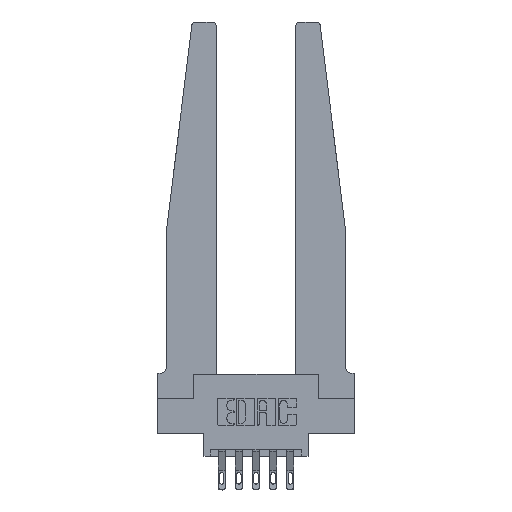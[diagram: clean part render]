
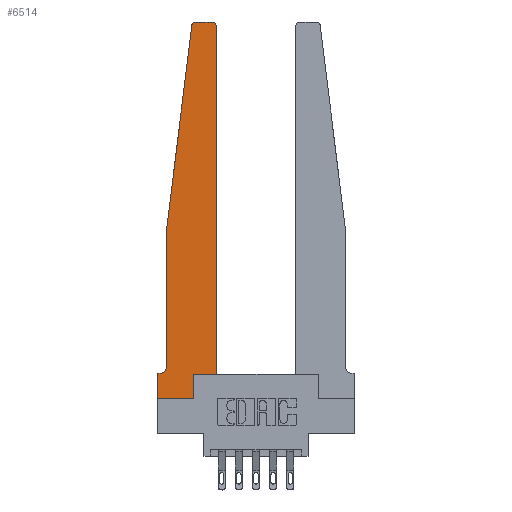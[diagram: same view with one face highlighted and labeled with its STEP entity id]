
A CAD part, top view. The second image highlights one B-rep face of the part: STEP entity #6514.
In plain terms, the highlighted planar face has unit normal (0, 0, 1).
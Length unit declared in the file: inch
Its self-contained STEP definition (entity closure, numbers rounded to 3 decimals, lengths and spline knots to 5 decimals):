
#19 = CARTESIAN_POINT ( 'NONE',  ( 0.015, 0.2375, 0.37 ) ) ;
#197 = CARTESIAN_POINT ( 'NONE',  ( 0.395, 2.72, 0.37 ) ) ;
#228 = DIRECTION ( 'NONE',  ( 0., 1., 0. ) ) ;
#386 = CARTESIAN_POINT ( 'NONE',  ( 0., 0., 0.37 ) ) ;
#636 = EDGE_CURVE ( 'NONE', #9752, #9828, #5890, .T. ) ;
#677 = ORIENTED_EDGE ( 'NONE', *, *, #7443, .T. ) ;
#765 = CARTESIAN_POINT ( 'NONE',  ( 0.015, 0.1875, 0.37 ) ) ;
#1002 = DIRECTION ( 'NONE',  ( 0., 0., 1. ) ) ;
#1082 = CARTESIAN_POINT ( 'NONE',  ( 0.395, 2.75, 0.37 ) ) ;
#1124 = DIRECTION ( 'NONE',  ( -1., 0., 0. ) ) ;
#1172 = ORIENTED_EDGE ( 'NONE', *, *, #7420, .T. ) ;
#1224 = EDGE_CURVE ( 'NONE', #6389, #5441, #4889, .T. ) ;
#1286 = CARTESIAN_POINT ( 'NONE',  ( 0., 0., 0.37 ) ) ;
#1292 = DIRECTION ( 'NONE',  ( 1., 0., 0. ) ) ;
#1352 = VERTEX_POINT ( 'NONE', #8733 ) ;
#1486 = DIRECTION ( 'NONE',  ( 1., 0., 0. ) ) ;
#1792 = DIRECTION ( 'NONE',  ( 0., 1., 0. ) ) ;
#1911 = CARTESIAN_POINT ( 'NONE',  ( 0.065, 1.25, 0.37 ) ) ;
#2294 = AXIS2_PLACEMENT_3D ( 'NONE', #197, #7592, #1292 ) ;
#2538 = EDGE_CURVE ( 'NONE', #5441, #6210, #10735, .T. ) ;
#2612 = ORIENTED_EDGE ( 'NONE', *, *, #3065, .T. ) ;
#2754 = EDGE_CURVE ( 'NONE', #3234, #9752, #9168, .T. ) ;
#2767 = LINE ( 'NONE', #7029, #10671 ) ;
#3065 = EDGE_CURVE ( 'NONE', #9119, #3821, #10401, .T. ) ;
#3234 = VERTEX_POINT ( 'NONE', #10200 ) ;
#3355 = ORIENTED_EDGE ( 'NONE', *, *, #2754, .T. ) ;
#3390 = EDGE_CURVE ( 'NONE', #9828, #6389, #12640, .T. ) ;
#3408 = CARTESIAN_POINT ( 'NONE',  ( 0.2605, 0., 0.37 ) ) ;
#3821 = VERTEX_POINT ( 'NONE', #11224 ) ;
#4039 = FACE_OUTER_BOUND ( 'NONE', #5125, .T. ) ;
#4076 = CARTESIAN_POINT ( 'NONE',  ( 0.425, 2.72, 0.37 ) ) ;
#4079 = EDGE_CURVE ( 'NONE', #6210, #12400, #5560, .T. ) ;
#4359 = LINE ( 'NONE', #11742, #9854 ) ;
#4742 = DIRECTION ( 'NONE',  ( 0., 0., 1. ) ) ;
#4889 = LINE ( 'NONE', #10332, #8630 ) ;
#5109 = EDGE_CURVE ( 'NONE', #12400, #1352, #2767, .T. ) ;
#5125 = EDGE_LOOP ( 'NONE', ( #2612, #677, #3355, #11997, #11505, #6135, #8378, #11215, #8584, #1172, #10811, #10345 ) ) ;
#5441 = VERTEX_POINT ( 'NONE', #12563 ) ;
#5560 = LINE ( 'NONE', #1286, #8004 ) ;
#5668 = CARTESIAN_POINT ( 'NONE',  ( 0.425, 0.18, 0.37 ) ) ;
#5679 = CARTESIAN_POINT ( 'NONE',  ( 0.25, 2.75, 0.37 ) ) ;
#5890 = LINE ( 'NONE', #6019, #11023 ) ;
#6019 = CARTESIAN_POINT ( 'NONE',  ( 0.065, 1.25, 0.37 ) ) ;
#6091 = VECTOR ( 'NONE', #12158, 39.37008 ) ;
#6135 = ORIENTED_EDGE ( 'NONE', *, *, #1224, .T. ) ;
#6210 = VERTEX_POINT ( 'NONE', #6862 ) ;
#6389 = VERTEX_POINT ( 'NONE', #765 ) ;
#6514 = ADVANCED_FACE ( 'NONE', ( #4039 ), #11381, .T. ) ;
#6636 = CARTESIAN_POINT ( 'NONE',  ( 0.065, 0.2375, 0.37 ) ) ;
#6706 = DIRECTION ( 'NONE',  ( -1., 0., 0. ) ) ;
#6743 = CARTESIAN_POINT ( 'NONE',  ( 0.425, 0.18, 0.37 ) ) ;
#6862 = CARTESIAN_POINT ( 'NONE',  ( 0., 0., 0.37 ) ) ;
#7029 = CARTESIAN_POINT ( 'NONE',  ( 0.2605, 0.18, 0.37 ) ) ;
#7103 = CIRCLE ( 'NONE', #7312, 0.03 ) ;
#7297 = CARTESIAN_POINT ( 'NONE',  ( 0., 0.1875, 0.37 ) ) ;
#7312 = AXIS2_PLACEMENT_3D ( 'NONE', #10901, #4742, #11934 ) ;
#7338 = DIRECTION ( 'NONE',  ( -1., 0., 0. ) ) ;
#7418 = DIRECTION ( 'NONE',  ( 0., 0., -1. ) ) ;
#7420 = EDGE_CURVE ( 'NONE', #1352, #11284, #12850, .T. ) ;
#7443 = EDGE_CURVE ( 'NONE', #3821, #3234, #7103, .T. ) ;
#7592 = DIRECTION ( 'NONE',  ( 0., 0., 1. ) ) ;
#8004 = VECTOR ( 'NONE', #12724, 39.37008 ) ;
#8045 = VECTOR ( 'NONE', #8821, 39.37008 ) ;
#8159 = DIRECTION ( 'NONE',  ( 0., -1., 0. ) ) ;
#8354 = DIRECTION ( 'NONE',  ( 1., 0., 0. ) ) ;
#8378 = ORIENTED_EDGE ( 'NONE', *, *, #2538, .T. ) ;
#8584 = ORIENTED_EDGE ( 'NONE', *, *, #5109, .T. ) ;
#8630 = VECTOR ( 'NONE', #7338, 39.37008 ) ;
#8645 = CARTESIAN_POINT ( 'NONE',  ( 0.065, 1.25, 0.37 ) ) ;
#8733 = CARTESIAN_POINT ( 'NONE',  ( 0.2605, 0.18, 0.37 ) ) ;
#8821 = DIRECTION ( 'NONE',  ( 0., -1., 0. ) ) ;
#9119 = VERTEX_POINT ( 'NONE', #1082 ) ;
#9168 = LINE ( 'NONE', #1911, #6091 ) ;
#9464 = AXIS2_PLACEMENT_3D ( 'NONE', #7297, #1002, #8354 ) ;
#9752 = VERTEX_POINT ( 'NONE', #8645 ) ;
#9818 = AXIS2_PLACEMENT_3D ( 'NONE', #19, #7418, #1124 ) ;
#9828 = VERTEX_POINT ( 'NONE', #6636 ) ;
#9854 = VECTOR ( 'NONE', #228, 39.37008 ) ;
#10144 = VECTOR ( 'NONE', #1486, 39.37008 ) ;
#10200 = CARTESIAN_POINT ( 'NONE',  ( 0.24675, 2.72367, 0.37 ) ) ;
#10332 = CARTESIAN_POINT ( 'NONE',  ( 0.065, 0.1875, 0.37 ) ) ;
#10345 = ORIENTED_EDGE ( 'NONE', *, *, #11850, .T. ) ;
#10401 = LINE ( 'NONE', #5679, #12801 ) ;
#10671 = VECTOR ( 'NONE', #1792, 39.37008 ) ;
#10735 = LINE ( 'NONE', #386, #8045 ) ;
#10811 = ORIENTED_EDGE ( 'NONE', *, *, #12492, .T. ) ;
#10901 = CARTESIAN_POINT ( 'NONE',  ( 0.27653, 2.72, 0.37 ) ) ;
#11023 = VECTOR ( 'NONE', #8159, 39.37008 ) ;
#11215 = ORIENTED_EDGE ( 'NONE', *, *, #4079, .T. ) ;
#11224 = CARTESIAN_POINT ( 'NONE',  ( 0.27653, 2.75, 0.37 ) ) ;
#11284 = VERTEX_POINT ( 'NONE', #5668 ) ;
#11287 = CIRCLE ( 'NONE', #2294, 0.03 ) ;
#11381 = PLANE ( 'NONE',  #9464 ) ;
#11505 = ORIENTED_EDGE ( 'NONE', *, *, #3390, .T. ) ;
#11742 = CARTESIAN_POINT ( 'NONE',  ( 0.425, 0.18, 0.37 ) ) ;
#11850 = EDGE_CURVE ( 'NONE', #12651, #9119, #11287, .T. ) ;
#11934 = DIRECTION ( 'NONE',  ( 1., 0., 0. ) ) ;
#11997 = ORIENTED_EDGE ( 'NONE', *, *, #636, .T. ) ;
#12158 = DIRECTION ( 'NONE',  ( -0.122, -0.992, 0. ) ) ;
#12400 = VERTEX_POINT ( 'NONE', #3408 ) ;
#12492 = EDGE_CURVE ( 'NONE', #11284, #12651, #4359, .T. ) ;
#12563 = CARTESIAN_POINT ( 'NONE',  ( 0., 0.1875, 0.37 ) ) ;
#12640 = CIRCLE ( 'NONE', #9818, 0.05 ) ;
#12651 = VERTEX_POINT ( 'NONE', #4076 ) ;
#12724 = DIRECTION ( 'NONE',  ( 1., 0., 0. ) ) ;
#12801 = VECTOR ( 'NONE', #6706, 39.37008 ) ;
#12850 = LINE ( 'NONE', #6743, #10144 ) ;
